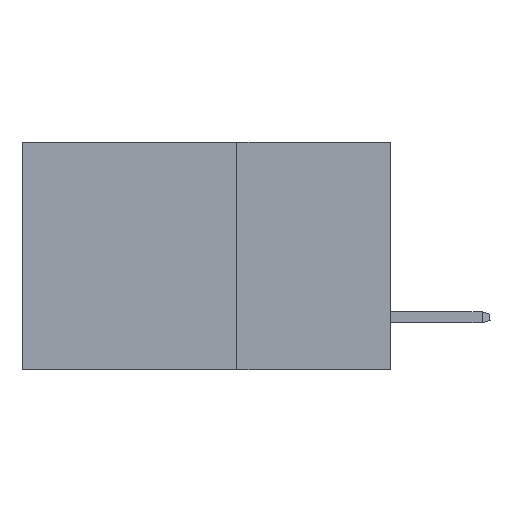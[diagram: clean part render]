
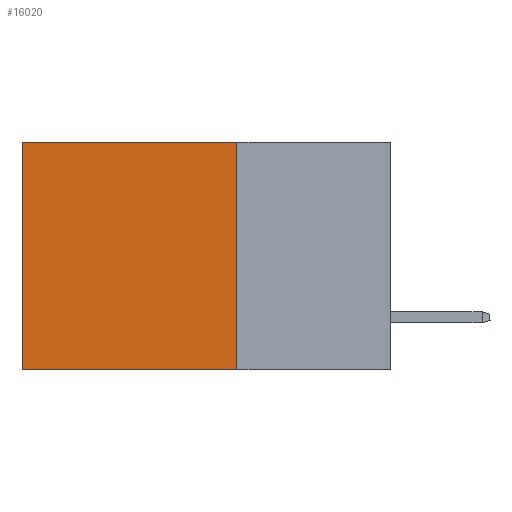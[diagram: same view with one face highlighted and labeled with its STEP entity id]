
A CAD part, left-side view. The second image highlights one B-rep face of the part: STEP entity #16020.
In plain terms, the highlighted planar face has unit normal (-1, 0, 0).
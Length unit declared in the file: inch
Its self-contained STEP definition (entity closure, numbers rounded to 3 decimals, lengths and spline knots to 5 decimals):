
#661 = EDGE_CURVE ( 'NONE', #10293, #11776, #16570, .T. ) ;
#732 = VECTOR ( 'NONE', #3254, 39.37008 ) ;
#1762 = AXIS2_PLACEMENT_3D ( 'NONE', #8640, #20029, #3847 ) ;
#2214 = EDGE_LOOP ( 'NONE', ( #6502, #15667, #19379, #10753 ) ) ;
#2476 = EDGE_CURVE ( 'NONE', #16398, #10293, #18774, .T. ) ;
#3254 = DIRECTION ( 'NONE',  ( 0., 1., 0. ) ) ;
#3267 = CARTESIAN_POINT ( 'NONE',  ( 0.2875, 0.25, 0. ) ) ;
#3847 = DIRECTION ( 'NONE',  ( 0., 0., -1. ) ) ;
#4772 = CARTESIAN_POINT ( 'NONE',  ( 0.2875, 0.6, -0.37 ) ) ;
#5351 = DIRECTION ( 'NONE',  ( 0., 0., -1. ) ) ;
#6490 = CARTESIAN_POINT ( 'NONE',  ( 0.2875, 0.6, 0. ) ) ;
#6502 = ORIENTED_EDGE ( 'NONE', *, *, #7123, .T. ) ;
#6722 = CARTESIAN_POINT ( 'NONE',  ( 0.2875, 0.25, -0.37 ) ) ;
#7041 = DIRECTION ( 'NONE',  ( 0., 1., 0. ) ) ;
#7123 = EDGE_CURVE ( 'NONE', #19272, #11776, #13756, .T. ) ;
#8640 = CARTESIAN_POINT ( 'NONE',  ( 0.2875, 0.25, 0. ) ) ;
#10293 = VERTEX_POINT ( 'NONE', #6722 ) ;
#10753 = ORIENTED_EDGE ( 'NONE', *, *, #18939, .T. ) ;
#11173 = CARTESIAN_POINT ( 'NONE',  ( 0.2875, 0.25, -0.37 ) ) ;
#11776 = VERTEX_POINT ( 'NONE', #4772 ) ;
#13448 = CARTESIAN_POINT ( 'NONE',  ( 0.2875, 0.25, 0. ) ) ;
#13756 = LINE ( 'NONE', #6490, #16587 ) ;
#14350 = CARTESIAN_POINT ( 'NONE',  ( 0.2875, 0.6, 0. ) ) ;
#14990 = VECTOR ( 'NONE', #7041, 39.37008 ) ;
#15174 = DIRECTION ( 'NONE',  ( 0., 0., -1. ) ) ;
#15667 = ORIENTED_EDGE ( 'NONE', *, *, #661, .F. ) ;
#16020 = ADVANCED_FACE ( 'NONE', ( #19188 ), #19886, .F. ) ;
#16398 = VERTEX_POINT ( 'NONE', #3267 ) ;
#16570 = LINE ( 'NONE', #11173, #732 ) ;
#16587 = VECTOR ( 'NONE', #5351, 39.37008 ) ;
#18436 = CARTESIAN_POINT ( 'NONE',  ( 0.2875, 0.25, 0. ) ) ;
#18516 = VECTOR ( 'NONE', #15174, 39.37008 ) ;
#18774 = LINE ( 'NONE', #13448, #18516 ) ;
#18939 = EDGE_CURVE ( 'NONE', #16398, #19272, #19348, .T. ) ;
#19188 = FACE_OUTER_BOUND ( 'NONE', #2214, .T. ) ;
#19272 = VERTEX_POINT ( 'NONE', #14350 ) ;
#19348 = LINE ( 'NONE', #18436, #14990 ) ;
#19379 = ORIENTED_EDGE ( 'NONE', *, *, #2476, .F. ) ;
#19886 = PLANE ( 'NONE',  #1762 ) ;
#20029 = DIRECTION ( 'NONE',  ( 1., 0., 0. ) ) ;
